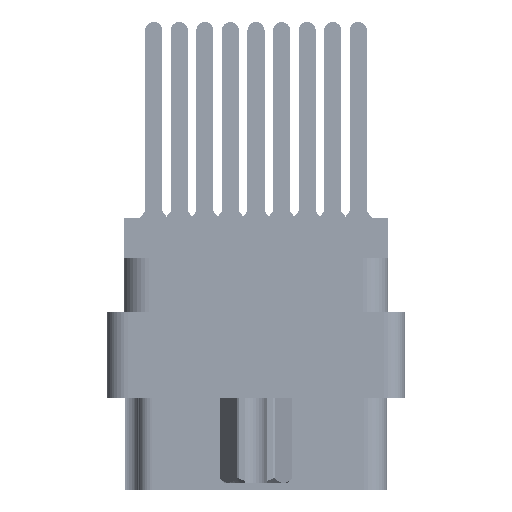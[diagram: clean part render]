
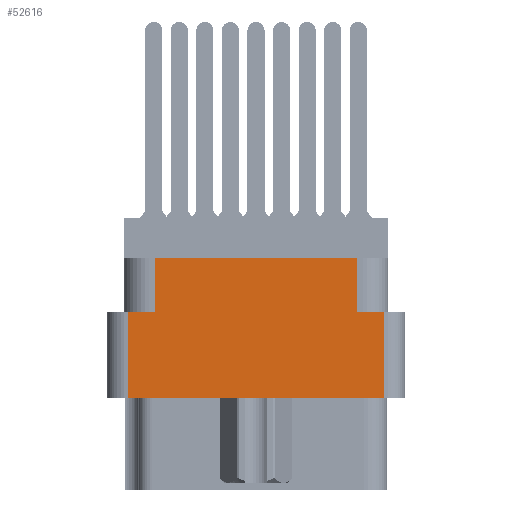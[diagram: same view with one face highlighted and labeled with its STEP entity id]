
A CAD part, left-side view. The second image highlights one B-rep face of the part: STEP entity #52616.
In plain terms, the highlighted planar face has unit normal (-1, 0, 0).
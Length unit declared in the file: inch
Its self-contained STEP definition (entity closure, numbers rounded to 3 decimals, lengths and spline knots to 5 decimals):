
#1019 = VERTEX_POINT ( 'NONE', #30057 ) ;
#1122 = VERTEX_POINT ( 'NONE', #16026 ) ;
#1609 = EDGE_CURVE ( 'NONE', #1019, #11986, #26311, .T. ) ;
#2354 = VECTOR ( 'NONE', #43050, 39.37008 ) ;
#2518 = LINE ( 'NONE', #5000, #27253 ) ;
#2876 = LINE ( 'NONE', #22217, #35537 ) ;
#5000 = CARTESIAN_POINT ( 'NONE',  ( -1.296, 0.438, -0.117 ) ) ;
#5448 = DIRECTION ( 'NONE',  ( 0., 0., 1. ) ) ;
#9534 = CARTESIAN_POINT ( 'NONE',  ( -1.296, -0.376, -0.529 ) ) ;
#10080 = CARTESIAN_POINT ( 'NONE',  ( -1.296, 0., -0.277 ) ) ;
#10086 = VERTEX_POINT ( 'NONE', #9534 ) ;
#11986 = VERTEX_POINT ( 'NONE', #58442 ) ;
#12256 = ORIENTED_EDGE ( 'NONE', *, *, #28062, .T. ) ;
#12956 = VECTOR ( 'NONE', #28988, 39.37008 ) ;
#13233 = CARTESIAN_POINT ( 'NONE',  ( -1.296, -0.376, -0.277 ) ) ;
#14756 = DIRECTION ( 'NONE',  ( 0., 0., -1. ) ) ;
#15632 = VECTOR ( 'NONE', #5448, 39.37008 ) ;
#16026 = CARTESIAN_POINT ( 'NONE',  ( -1.296, 0.376, -0.529 ) ) ;
#16498 = DIRECTION ( 'NONE',  ( 0., 0., 1. ) ) ;
#17973 = ORIENTED_EDGE ( 'NONE', *, *, #30588, .F. ) ;
#18513 = EDGE_CURVE ( 'NONE', #23443, #26206, #2518, .T. ) ;
#19471 = CARTESIAN_POINT ( 'NONE',  ( -1.296, 0., -0.277 ) ) ;
#19802 = CARTESIAN_POINT ( 'NONE',  ( -1.296, -0.296, -0.277 ) ) ;
#20684 = ORIENTED_EDGE ( 'NONE', *, *, #25436, .F. ) ;
#21357 = EDGE_CURVE ( 'NONE', #10086, #55477, #43626, .T. ) ;
#22217 = CARTESIAN_POINT ( 'NONE',  ( -1.296, 0., -0.529 ) ) ;
#23114 = DIRECTION ( 'NONE',  ( 0., 0., 1. ) ) ;
#23228 = DIRECTION ( 'NONE',  ( 0., 0., 1. ) ) ;
#23443 = VERTEX_POINT ( 'NONE', #33046 ) ;
#24560 = LINE ( 'NONE', #10080, #12956 ) ;
#25385 = ORIENTED_EDGE ( 'NONE', *, *, #18513, .F. ) ;
#25415 = EDGE_LOOP ( 'NONE', ( #39649, #33200, #17973, #41084, #34395, #12256, #25385, #20684 ) ) ;
#25436 = EDGE_CURVE ( 'NONE', #11986, #23443, #38955, .T. ) ;
#26044 = PLANE ( 'NONE',  #51024 ) ;
#26206 = VERTEX_POINT ( 'NONE', #27281 ) ;
#26311 = LINE ( 'NONE', #19471, #2354 ) ;
#27087 = DIRECTION ( 'NONE',  ( 0., 1., 0. ) ) ;
#27253 = VECTOR ( 'NONE', #27701, 39.37008 ) ;
#27281 = CARTESIAN_POINT ( 'NONE',  ( -1.296, -0.296, -0.117 ) ) ;
#27701 = DIRECTION ( 'NONE',  ( 0., -1., 0. ) ) ;
#28062 = EDGE_CURVE ( 'NONE', #36780, #26206, #48788, .T. ) ;
#28988 = DIRECTION ( 'NONE',  ( 0., -1., 0. ) ) ;
#29206 = CARTESIAN_POINT ( 'NONE',  ( -1.296, 0.376, -0.798 ) ) ;
#30057 = CARTESIAN_POINT ( 'NONE',  ( -1.296, 0.376, -0.277 ) ) ;
#30588 = EDGE_CURVE ( 'NONE', #10086, #1122, #2876, .T. ) ;
#33046 = CARTESIAN_POINT ( 'NONE',  ( -1.296, 0.296, -0.117 ) ) ;
#33200 = ORIENTED_EDGE ( 'NONE', *, *, #42540, .T. ) ;
#34395 = ORIENTED_EDGE ( 'NONE', *, *, #46682, .F. ) ;
#34614 = CARTESIAN_POINT ( 'NONE',  ( -1.296, -0.438, -0.798 ) ) ;
#35537 = VECTOR ( 'NONE', #27087, 39.37008 ) ;
#36780 = VERTEX_POINT ( 'NONE', #45173 ) ;
#38033 = VECTOR ( 'NONE', #14756, 39.37008 ) ;
#38685 = FACE_OUTER_BOUND ( 'NONE', #25415, .T. ) ;
#38955 = LINE ( 'NONE', #55662, #15632 ) ;
#39267 = VECTOR ( 'NONE', #23114, 39.37008 ) ;
#39649 = ORIENTED_EDGE ( 'NONE', *, *, #1609, .F. ) ;
#40925 = LINE ( 'NONE', #29206, #38033 ) ;
#41084 = ORIENTED_EDGE ( 'NONE', *, *, #21357, .T. ) ;
#42540 = EDGE_CURVE ( 'NONE', #1019, #1122, #40925, .T. ) ;
#43050 = DIRECTION ( 'NONE',  ( 0., -1., 0. ) ) ;
#43626 = LINE ( 'NONE', #46228, #39267 ) ;
#45173 = CARTESIAN_POINT ( 'NONE',  ( -1.296, -0.296, -0.277 ) ) ;
#46228 = CARTESIAN_POINT ( 'NONE',  ( -1.296, -0.376, -0.798 ) ) ;
#46334 = DIRECTION ( 'NONE',  ( -1., 0., 0. ) ) ;
#46682 = EDGE_CURVE ( 'NONE', #36780, #55477, #24560, .T. ) ;
#48788 = LINE ( 'NONE', #19802, #49545 ) ;
#49545 = VECTOR ( 'NONE', #16498, 39.37008 ) ;
#51024 = AXIS2_PLACEMENT_3D ( 'NONE', #34614, #46334, #23228 ) ;
#52616 = ADVANCED_FACE ( 'NONE', ( #38685 ), #26044, .T. ) ;
#55477 = VERTEX_POINT ( 'NONE', #13233 ) ;
#55662 = CARTESIAN_POINT ( 'NONE',  ( -1.296, 0.296, -0.277 ) ) ;
#58442 = CARTESIAN_POINT ( 'NONE',  ( -1.296, 0.296, -0.277 ) ) ;
